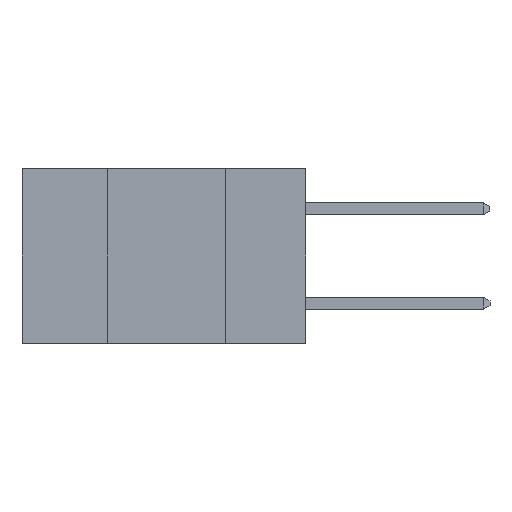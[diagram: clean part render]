
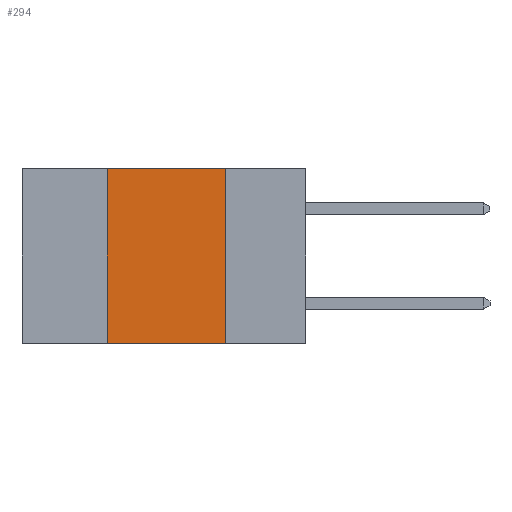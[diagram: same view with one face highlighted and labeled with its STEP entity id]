
A CAD part, left-side view. The second image highlights one B-rep face of the part: STEP entity #294.
In plain terms, the highlighted planar face has unit normal (-1, 0, 0).
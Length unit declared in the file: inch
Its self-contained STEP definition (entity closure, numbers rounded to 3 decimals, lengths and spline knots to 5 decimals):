
#111 = AXIS2_PLACEMENT_3D ( 'NONE', #4121, #5722, #2712 ) ;
#294 = ADVANCED_FACE ( 'NONE', ( #5978 ), #4285, .F. ) ;
#313 = CARTESIAN_POINT ( 'NONE',  ( 0., 0.17, -0.37 ) ) ;
#405 = EDGE_CURVE ( 'NONE', #1702, #5372, #4881, .T. ) ;
#1143 = ORIENTED_EDGE ( 'NONE', *, *, #7694, .F. ) ;
#1154 = ORIENTED_EDGE ( 'NONE', *, *, #5118, .F. ) ;
#1170 = ORIENTED_EDGE ( 'NONE', *, *, #2848, .F. ) ;
#1191 = ORIENTED_EDGE ( 'NONE', *, *, #405, .T. ) ;
#1325 = EDGE_LOOP ( 'NONE', ( #1143, #1154, #1170, #1191 ) ) ;
#1702 = VERTEX_POINT ( 'NONE', #7620 ) ;
#2501 = CARTESIAN_POINT ( 'NONE',  ( 0., 0.17, 0. ) ) ;
#2712 = DIRECTION ( 'NONE',  ( 0., 0., -1. ) ) ;
#2848 = EDGE_CURVE ( 'NONE', #1702, #7116, #5769, .T. ) ;
#3046 = CARTESIAN_POINT ( 'NONE',  ( 0., 0.6, 0. ) ) ;
#3100 = VECTOR ( 'NONE', #5435, 39.37008 ) ;
#3113 = DIRECTION ( 'NONE',  ( 0., -1., 0. ) ) ;
#3125 = LINE ( 'NONE', #5110, #8105 ) ;
#3216 = CARTESIAN_POINT ( 'NONE',  ( 0., 0.6, -0.37 ) ) ;
#4121 = CARTESIAN_POINT ( 'NONE',  ( 0., 0.6, 0. ) ) ;
#4285 = PLANE ( 'NONE',  #111 ) ;
#4536 = CARTESIAN_POINT ( 'NONE',  ( 0., 0.42, -0.37 ) ) ;
#4546 = DIRECTION ( 'NONE',  ( 0., 0., 1. ) ) ;
#4881 = LINE ( 'NONE', #3216, #3100 ) ;
#4947 = LINE ( 'NONE', #3046, #8132 ) ;
#5101 = DIRECTION ( 'NONE',  ( 0., 0., -1. ) ) ;
#5110 = CARTESIAN_POINT ( 'NONE',  ( 0., 0.17, -0.37 ) ) ;
#5118 = EDGE_CURVE ( 'NONE', #7116, #5139, #4947, .T. ) ;
#5139 = VERTEX_POINT ( 'NONE', #2501 ) ;
#5372 = VERTEX_POINT ( 'NONE', #313 ) ;
#5435 = DIRECTION ( 'NONE',  ( 0., -1., 0. ) ) ;
#5568 = VECTOR ( 'NONE', #4546, 39.37008 ) ;
#5722 = DIRECTION ( 'NONE',  ( 1., 0., 0. ) ) ;
#5769 = LINE ( 'NONE', #4536, #5568 ) ;
#5978 = FACE_OUTER_BOUND ( 'NONE', #1325, .T. ) ;
#6195 = CARTESIAN_POINT ( 'NONE',  ( 0., 0.42, 0. ) ) ;
#7116 = VERTEX_POINT ( 'NONE', #6195 ) ;
#7620 = CARTESIAN_POINT ( 'NONE',  ( 0., 0.42, -0.37 ) ) ;
#7694 = EDGE_CURVE ( 'NONE', #5139, #5372, #3125, .T. ) ;
#8105 = VECTOR ( 'NONE', #5101, 39.37008 ) ;
#8132 = VECTOR ( 'NONE', #3113, 39.37008 ) ;
